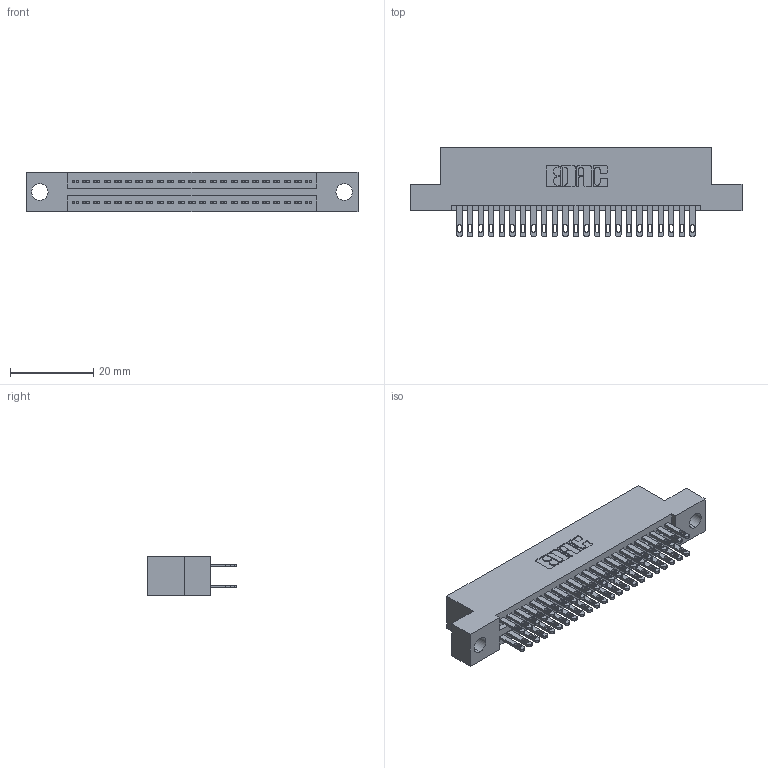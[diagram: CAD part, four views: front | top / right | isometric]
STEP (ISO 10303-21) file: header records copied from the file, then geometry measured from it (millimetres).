
FILE_DESCRIPTION (( 'STEP AP203' ), '1' );
FILE_NAME ('345-046-500-204.STEP', '2021-05-20T02:11:54', ( '' ), ( '' ), 'SwSTEP 2.0', 'SolidWorks 2020', '' );
FILE_SCHEMA (( 'CONFIG_CONTROL_DESIGN' ));
Length unit declared in the file: inch
Products named in the file (3): 345 Part_Flush Mounting Lugs - 0.156 Dia-TI; 345-046-500-204; 345-292-001_345-293-100
Assembly tree (47 placements, depth 2):
  345-046-500-204
    345 Part_Flush Mounting Lugs - 0.156 Dia-TI
    345-292-001_345-293-100  x46
Bounding box: 79.63 x 21.51 x 9.4 mm (x, y, z)
Volume: 7593.5 mm3; surface area: 11177.2 mm2
Topology: 47 solids, 47 shells, 2256 faces, 6863 edges, 4574 vertices
Faces by surface type: plane 1336, cylinder 920
Entity records: 20953 total; most frequent: CARTESIAN_POINT 3534, ORIENTED_EDGE 3466, DIRECTION 3141, EDGE_CURVE 1733, LINE 1505, VECTOR 1505, VERTEX_POINT 1154, AXIS2_PLACEMENT_3D 818
